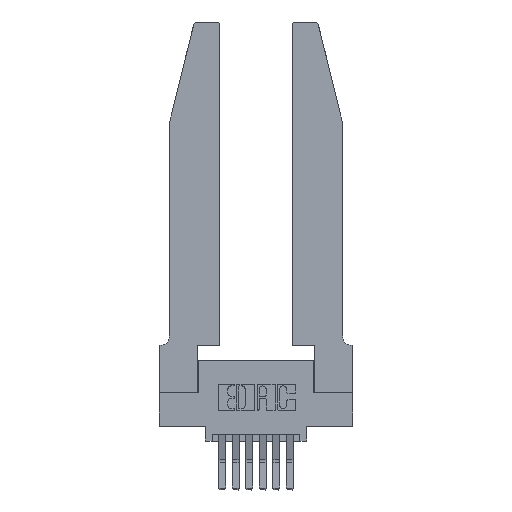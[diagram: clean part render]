
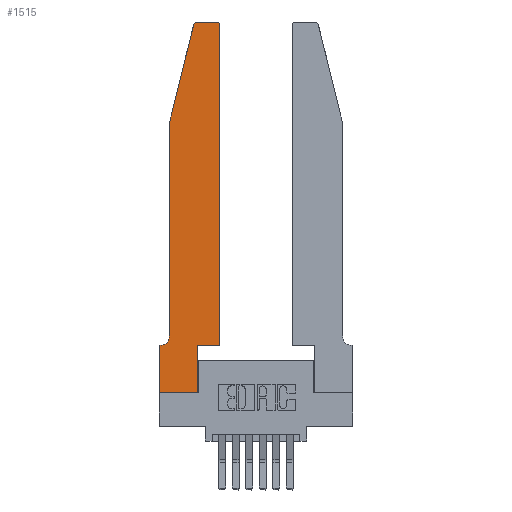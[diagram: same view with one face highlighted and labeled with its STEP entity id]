
A CAD part, top view. The second image highlights one B-rep face of the part: STEP entity #1515.
In plain terms, the highlighted planar face has unit normal (0, 0, 1).
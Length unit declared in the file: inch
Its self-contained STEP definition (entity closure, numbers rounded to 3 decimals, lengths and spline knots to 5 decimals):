
#34 = AXIS2_PLACEMENT_3D ( 'NONE', #4994, #11807, #10685 ) ;
#623 = DIRECTION ( 'NONE',  ( 1., 0., 0. ) ) ;
#634 = DIRECTION ( 'NONE',  ( 0., -1., 0. ) ) ;
#830 = CARTESIAN_POINT ( 'NONE',  ( 0.25487, 2.72718, 0.37 ) ) ;
#862 = DIRECTION ( 'NONE',  ( 1., 0., 0. ) ) ;
#987 = DIRECTION ( 'NONE',  ( 0., 0., -1. ) ) ;
#1428 = VERTEX_POINT ( 'NONE', #9493 ) ;
#1506 = ORIENTED_EDGE ( 'NONE', *, *, #13550, .T. ) ;
#1515 = ADVANCED_FACE ( 'NONE', ( #11251 ), #8349, .T. ) ;
#1644 = CARTESIAN_POINT ( 'NONE',  ( 0.0755, 0.35, 0.37 ) ) ;
#2064 = DIRECTION ( 'NONE',  ( 0., 0., 1. ) ) ;
#2105 = VERTEX_POINT ( 'NONE', #3694 ) ;
#2112 = EDGE_CURVE ( 'NONE', #3983, #2105, #10354, .T. ) ;
#2277 = LINE ( 'NONE', #13642, #11437 ) ;
#2435 = EDGE_CURVE ( 'NONE', #10074, #8313, #11044, .T. ) ;
#2662 = VERTEX_POINT ( 'NONE', #9358 ) ;
#2684 = VECTOR ( 'NONE', #862, 39.37008 ) ;
#2740 = CARTESIAN_POINT ( 'NONE',  ( 0.0755, 2., 0.37 ) ) ;
#3089 = CARTESIAN_POINT ( 'NONE',  ( 0.284, 2.75, 0.37 ) ) ;
#3345 = DIRECTION ( 'NONE',  ( -1., 0., 0. ) ) ;
#3694 = CARTESIAN_POINT ( 'NONE',  ( 0.0755, 2., 0.37 ) ) ;
#3740 = CARTESIAN_POINT ( 'NONE',  ( 0.0055, 0.35, 0.37 ) ) ;
#3861 = VERTEX_POINT ( 'NONE', #4660 ) ;
#3983 = VERTEX_POINT ( 'NONE', #830 ) ;
#4627 = VECTOR ( 'NONE', #5476, 39.37008 ) ;
#4660 = CARTESIAN_POINT ( 'NONE',  ( 0.0755, 0.42, 0.37 ) ) ;
#4792 = LINE ( 'NONE', #1644, #13920 ) ;
#4994 = CARTESIAN_POINT ( 'NONE',  ( 0., 0.35, 0.37 ) ) ;
#4995 = VECTOR ( 'NONE', #634, 39.37008 ) ;
#5217 = EDGE_CURVE ( 'NONE', #9277, #2662, #8174, .T. ) ;
#5265 = ORIENTED_EDGE ( 'NONE', *, *, #10955, .T. ) ;
#5310 = DIRECTION ( 'NONE',  ( -1., 0., 0. ) ) ;
#5321 = CARTESIAN_POINT ( 'NONE',  ( 0.2865, 0., 0.37 ) ) ;
#5379 = CARTESIAN_POINT ( 'NONE',  ( 0., 0., 0.37 ) ) ;
#5476 = DIRECTION ( 'NONE',  ( 0., 1., 0. ) ) ;
#5792 = VECTOR ( 'NONE', #6586, 39.37008 ) ;
#5986 = AXIS2_PLACEMENT_3D ( 'NONE', #8894, #987, #3345 ) ;
#6088 = ORIENTED_EDGE ( 'NONE', *, *, #8711, .T. ) ;
#6470 = EDGE_CURVE ( 'NONE', #12957, #3983, #9243, .T. ) ;
#6475 = ORIENTED_EDGE ( 'NONE', *, *, #2112, .T. ) ;
#6486 = VECTOR ( 'NONE', #11548, 39.37008 ) ;
#6564 = VERTEX_POINT ( 'NONE', #13167 ) ;
#6586 = DIRECTION ( 'NONE',  ( 0., -1., 0. ) ) ;
#6656 = CARTESIAN_POINT ( 'NONE',  ( 0.4505, 0.35, 0.37 ) ) ;
#7109 = AXIS2_PLACEMENT_3D ( 'NONE', #13292, #2064, #8858 ) ;
#7280 = ORIENTED_EDGE ( 'NONE', *, *, #13983, .T. ) ;
#7482 = CARTESIAN_POINT ( 'NONE',  ( 0.284, 2.72, 0.37 ) ) ;
#7517 = ORIENTED_EDGE ( 'NONE', *, *, #8004, .T. ) ;
#7866 = CARTESIAN_POINT ( 'NONE',  ( 0.4505, 0.35, 0.37 ) ) ;
#7867 = CIRCLE ( 'NONE', #5986, 0.07 ) ;
#8004 = EDGE_CURVE ( 'NONE', #14225, #1428, #12162, .T. ) ;
#8141 = ORIENTED_EDGE ( 'NONE', *, *, #5217, .T. ) ;
#8174 = LINE ( 'NONE', #12939, #4995 ) ;
#8255 = LINE ( 'NONE', #9975, #5792 ) ;
#8313 = VERTEX_POINT ( 'NONE', #9236 ) ;
#8349 = PLANE ( 'NONE',  #34 ) ;
#8711 = EDGE_CURVE ( 'NONE', #2662, #10074, #14091, .T. ) ;
#8858 = DIRECTION ( 'NONE',  ( 1., 0., 0. ) ) ;
#8894 = CARTESIAN_POINT ( 'NONE',  ( 0.0055, 0.42, 0.37 ) ) ;
#9236 = CARTESIAN_POINT ( 'NONE',  ( 0.2865, 0.35, 0.37 ) ) ;
#9243 = CIRCLE ( 'NONE', #9794, 0.03 ) ;
#9277 = VERTEX_POINT ( 'NONE', #11259 ) ;
#9294 = EDGE_CURVE ( 'NONE', #1428, #6564, #13021, .T. ) ;
#9358 = CARTESIAN_POINT ( 'NONE',  ( 0., 0., 0.37 ) ) ;
#9493 = CARTESIAN_POINT ( 'NONE',  ( 0.4505, 2.72, 0.37 ) ) ;
#9561 = LINE ( 'NONE', #6656, #13378 ) ;
#9608 = ORIENTED_EDGE ( 'NONE', *, *, #9294, .T. ) ;
#9794 = AXIS2_PLACEMENT_3D ( 'NONE', #7482, #10893, #623 ) ;
#9975 = CARTESIAN_POINT ( 'NONE',  ( 0.0755, 2., 0.37 ) ) ;
#10074 = VERTEX_POINT ( 'NONE', #5321 ) ;
#10155 = ORIENTED_EDGE ( 'NONE', *, *, #12385, .T. ) ;
#10238 = DIRECTION ( 'NONE',  ( -1., 0., 0. ) ) ;
#10275 = EDGE_CURVE ( 'NONE', #6564, #12957, #2277, .T. ) ;
#10354 = LINE ( 'NONE', #2740, #6486 ) ;
#10685 = DIRECTION ( 'NONE',  ( 1., 0., 0. ) ) ;
#10893 = DIRECTION ( 'NONE',  ( 0., 0., 1. ) ) ;
#10955 = EDGE_CURVE ( 'NONE', #2105, #3861, #8255, .T. ) ;
#11003 = EDGE_LOOP ( 'NONE', ( #13112, #11641, #6475, #5265, #10155, #7280, #8141, #6088, #14395, #1506, #7517, #9608 ) ) ;
#11044 = LINE ( 'NONE', #14038, #13472 ) ;
#11179 = DIRECTION ( 'NONE',  ( 1., 0., 0. ) ) ;
#11251 = FACE_OUTER_BOUND ( 'NONE', #11003, .T. ) ;
#11259 = CARTESIAN_POINT ( 'NONE',  ( 0., 0.35, 0.37 ) ) ;
#11437 = VECTOR ( 'NONE', #10238, 39.37008 ) ;
#11548 = DIRECTION ( 'NONE',  ( -0.239, -0.971, 0. ) ) ;
#11641 = ORIENTED_EDGE ( 'NONE', *, *, #6470, .T. ) ;
#11807 = DIRECTION ( 'NONE',  ( 0., 0., 1. ) ) ;
#12162 = LINE ( 'NONE', #14408, #4627 ) ;
#12385 = EDGE_CURVE ( 'NONE', #3861, #12990, #7867, .T. ) ;
#12939 = CARTESIAN_POINT ( 'NONE',  ( 0., 0., 0.37 ) ) ;
#12957 = VERTEX_POINT ( 'NONE', #3089 ) ;
#12990 = VERTEX_POINT ( 'NONE', #3740 ) ;
#13021 = CIRCLE ( 'NONE', #7109, 0.03 ) ;
#13112 = ORIENTED_EDGE ( 'NONE', *, *, #10275, .T. ) ;
#13167 = CARTESIAN_POINT ( 'NONE',  ( 0.4205, 2.75, 0.37 ) ) ;
#13292 = CARTESIAN_POINT ( 'NONE',  ( 0.4205, 2.72, 0.37 ) ) ;
#13378 = VECTOR ( 'NONE', #11179, 39.37008 ) ;
#13472 = VECTOR ( 'NONE', #14182, 39.37008 ) ;
#13550 = EDGE_CURVE ( 'NONE', #8313, #14225, #9561, .T. ) ;
#13642 = CARTESIAN_POINT ( 'NONE',  ( 0.2605, 2.75, 0.37 ) ) ;
#13920 = VECTOR ( 'NONE', #5310, 39.37008 ) ;
#13983 = EDGE_CURVE ( 'NONE', #12990, #9277, #4792, .T. ) ;
#14038 = CARTESIAN_POINT ( 'NONE',  ( 0.2865, 0.35, 0.37 ) ) ;
#14091 = LINE ( 'NONE', #5379, #2684 ) ;
#14182 = DIRECTION ( 'NONE',  ( 0., 1., 0. ) ) ;
#14225 = VERTEX_POINT ( 'NONE', #7866 ) ;
#14395 = ORIENTED_EDGE ( 'NONE', *, *, #2435, .T. ) ;
#14408 = CARTESIAN_POINT ( 'NONE',  ( 0.4505, 0.35, 0.37 ) ) ;
